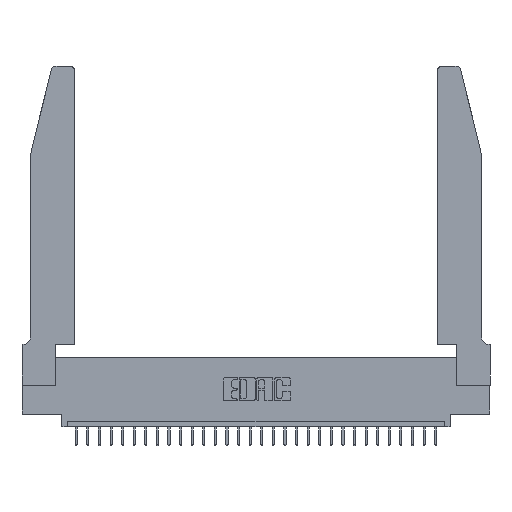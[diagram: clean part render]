
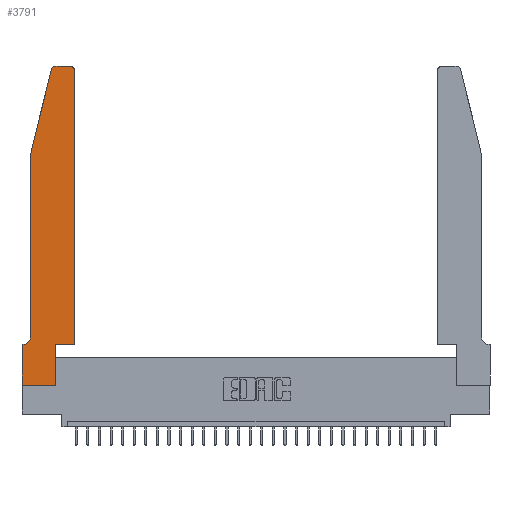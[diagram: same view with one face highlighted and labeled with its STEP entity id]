
A CAD part, top view. The second image highlights one B-rep face of the part: STEP entity #3791.
In plain terms, the highlighted planar face has unit normal (0, 0, 1).
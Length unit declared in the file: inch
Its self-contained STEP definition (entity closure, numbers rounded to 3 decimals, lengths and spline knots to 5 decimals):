
#134 = VECTOR ( 'NONE', #1609, 39.37008 ) ;
#528 = DIRECTION ( 'NONE',  ( 0., 0., 1. ) ) ;
#985 = DIRECTION ( 'NONE',  ( -1., 0., 0. ) ) ;
#990 = ORIENTED_EDGE ( 'NONE', *, *, #5058, .T. ) ;
#1609 = DIRECTION ( 'NONE',  ( 1., 0., 0. ) ) ;
#1809 = VECTOR ( 'NONE', #11846, 39.37008 ) ;
#2272 = EDGE_CURVE ( 'NONE', #11705, #8610, #29116, .T. ) ;
#2925 = VECTOR ( 'NONE', #13264, 39.37008 ) ;
#3066 = VECTOR ( 'NONE', #985, 39.37008 ) ;
#3258 = VERTEX_POINT ( 'NONE', #20159 ) ;
#3511 = ORIENTED_EDGE ( 'NONE', *, *, #26599, .T. ) ;
#3589 = ORIENTED_EDGE ( 'NONE', *, *, #25843, .T. ) ;
#3628 = EDGE_CURVE ( 'NONE', #18461, #7957, #4170, .T. ) ;
#3791 = ADVANCED_FACE ( 'NONE', ( #6734 ), #9200, .T. ) ;
#4170 = LINE ( 'NONE', #5717, #134 ) ;
#4307 = VECTOR ( 'NONE', #5583, 39.37008 ) ;
#5058 = EDGE_CURVE ( 'NONE', #7957, #29282, #20505, .T. ) ;
#5583 = DIRECTION ( 'NONE',  ( 0., -1., 0. ) ) ;
#5599 = EDGE_CURVE ( 'NONE', #6334, #9313, #20091, .T. ) ;
#5654 = DIRECTION ( 'NONE',  ( 0., 1., 0. ) ) ;
#5717 = CARTESIAN_POINT ( 'NONE',  ( 0.4505, 0.35, 0.37 ) ) ;
#6334 = VERTEX_POINT ( 'NONE', #29637 ) ;
#6403 = CARTESIAN_POINT ( 'NONE',  ( 0.0755, 2., 0.37 ) ) ;
#6659 = EDGE_CURVE ( 'NONE', #3258, #16181, #11992, .T. ) ;
#6734 = FACE_OUTER_BOUND ( 'NONE', #21080, .T. ) ;
#7278 = DIRECTION ( 'NONE',  ( 0., 0., -1. ) ) ;
#7701 = CARTESIAN_POINT ( 'NONE',  ( 0.0055, 0.42, 0.37 ) ) ;
#7957 = VERTEX_POINT ( 'NONE', #18358 ) ;
#8610 = VERTEX_POINT ( 'NONE', #6403 ) ;
#8666 = ORIENTED_EDGE ( 'NONE', *, *, #18599, .T. ) ;
#8841 = CARTESIAN_POINT ( 'NONE',  ( 0.0755, 2., 0.37 ) ) ;
#8984 = CARTESIAN_POINT ( 'NONE',  ( 0.4505, 2.72, 0.37 ) ) ;
#9177 = ORIENTED_EDGE ( 'NONE', *, *, #10182, .T. ) ;
#9200 = PLANE ( 'NONE',  #27149 ) ;
#9276 = DIRECTION ( 'NONE',  ( -0.239, -0.971, 0. ) ) ;
#9313 = VERTEX_POINT ( 'NONE', #20942 ) ;
#10182 = EDGE_CURVE ( 'NONE', #17042, #10856, #27306, .T. ) ;
#10247 = LINE ( 'NONE', #25930, #1809 ) ;
#10289 = CARTESIAN_POINT ( 'NONE',  ( 0., 0., 0.37 ) ) ;
#10739 = CARTESIAN_POINT ( 'NONE',  ( 0.284, 2.75, 0.37 ) ) ;
#10856 = VERTEX_POINT ( 'NONE', #10739 ) ;
#11136 = AXIS2_PLACEMENT_3D ( 'NONE', #26828, #24238, #19478 ) ;
#11151 = VECTOR ( 'NONE', #14341, 39.37008 ) ;
#11296 = VERTEX_POINT ( 'NONE', #16465 ) ;
#11705 = VERTEX_POINT ( 'NONE', #14014 ) ;
#11846 = DIRECTION ( 'NONE',  ( 0., 1., 0. ) ) ;
#11992 = CIRCLE ( 'NONE', #22037, 0.07 ) ;
#12599 = ORIENTED_EDGE ( 'NONE', *, *, #22833, .T. ) ;
#12634 = ORIENTED_EDGE ( 'NONE', *, *, #19811, .T. ) ;
#13264 = DIRECTION ( 'NONE',  ( 1., 0., 0. ) ) ;
#13458 = ORIENTED_EDGE ( 'NONE', *, *, #6659, .T. ) ;
#14014 = CARTESIAN_POINT ( 'NONE',  ( 0.25487, 2.72718, 0.37 ) ) ;
#14341 = DIRECTION ( 'NONE',  ( -1., 0., 0. ) ) ;
#14538 = CARTESIAN_POINT ( 'NONE',  ( 0.284, 2.72, 0.37 ) ) ;
#15014 = AXIS2_PLACEMENT_3D ( 'NONE', #14538, #528, #16856 ) ;
#15079 = CARTESIAN_POINT ( 'NONE',  ( 0.0755, 0.35, 0.37 ) ) ;
#15454 = DIRECTION ( 'NONE',  ( 0., -1., 0. ) ) ;
#16181 = VERTEX_POINT ( 'NONE', #18975 ) ;
#16263 = DIRECTION ( 'NONE',  ( -1., 0., 0. ) ) ;
#16465 = CARTESIAN_POINT ( 'NONE',  ( 0., 0.35, 0.37 ) ) ;
#16856 = DIRECTION ( 'NONE',  ( 1., 0., 0. ) ) ;
#17042 = VERTEX_POINT ( 'NONE', #28911 ) ;
#17098 = ORIENTED_EDGE ( 'NONE', *, *, #2272, .T. ) ;
#17205 = VECTOR ( 'NONE', #5654, 39.37008 ) ;
#17458 = ORIENTED_EDGE ( 'NONE', *, *, #5599, .T. ) ;
#17671 = LINE ( 'NONE', #15079, #3066 ) ;
#18071 = CIRCLE ( 'NONE', #15014, 0.03 ) ;
#18225 = ORIENTED_EDGE ( 'NONE', *, *, #21415, .T. ) ;
#18358 = CARTESIAN_POINT ( 'NONE',  ( 0.4505, 0.35, 0.37 ) ) ;
#18461 = VERTEX_POINT ( 'NONE', #21506 ) ;
#18599 = EDGE_CURVE ( 'NONE', #11296, #6334, #20736, .T. ) ;
#18975 = CARTESIAN_POINT ( 'NONE',  ( 0.0055, 0.35, 0.37 ) ) ;
#19478 = DIRECTION ( 'NONE',  ( 1., 0., 0. ) ) ;
#19811 = EDGE_CURVE ( 'NONE', #10856, #11705, #18071, .T. ) ;
#20091 = LINE ( 'NONE', #27334, #2925 ) ;
#20159 = CARTESIAN_POINT ( 'NONE',  ( 0.0755, 0.42, 0.37 ) ) ;
#20505 = LINE ( 'NONE', #24992, #17205 ) ;
#20736 = LINE ( 'NONE', #10289, #4307 ) ;
#20942 = CARTESIAN_POINT ( 'NONE',  ( 0.2865, 0., 0.37 ) ) ;
#21080 = EDGE_LOOP ( 'NONE', ( #9177, #12634, #17098, #3589, #13458, #3511, #8666, #17458, #12599, #23591, #990, #18225 ) ) ;
#21415 = EDGE_CURVE ( 'NONE', #29282, #17042, #22825, .T. ) ;
#21506 = CARTESIAN_POINT ( 'NONE',  ( 0.2865, 0.35, 0.37 ) ) ;
#22037 = AXIS2_PLACEMENT_3D ( 'NONE', #7701, #7278, #16263 ) ;
#22543 = LINE ( 'NONE', #8841, #26603 ) ;
#22825 = CIRCLE ( 'NONE', #11136, 0.03 ) ;
#22833 = EDGE_CURVE ( 'NONE', #9313, #18461, #10247, .T. ) ;
#22835 = VECTOR ( 'NONE', #9276, 39.37008 ) ;
#23591 = ORIENTED_EDGE ( 'NONE', *, *, #3628, .T. ) ;
#24238 = DIRECTION ( 'NONE',  ( 0., 0., 1. ) ) ;
#24992 = CARTESIAN_POINT ( 'NONE',  ( 0.4505, 0.35, 0.37 ) ) ;
#25791 = CARTESIAN_POINT ( 'NONE',  ( 0., 0.35, 0.37 ) ) ;
#25843 = EDGE_CURVE ( 'NONE', #8610, #3258, #22543, .T. ) ;
#25930 = CARTESIAN_POINT ( 'NONE',  ( 0.2865, 0.35, 0.37 ) ) ;
#26599 = EDGE_CURVE ( 'NONE', #16181, #11296, #17671, .T. ) ;
#26603 = VECTOR ( 'NONE', #15454, 39.37008 ) ;
#26828 = CARTESIAN_POINT ( 'NONE',  ( 0.4205, 2.72, 0.37 ) ) ;
#27149 = AXIS2_PLACEMENT_3D ( 'NONE', #25791, #30416, #27842 ) ;
#27306 = LINE ( 'NONE', #28437, #11151 ) ;
#27334 = CARTESIAN_POINT ( 'NONE',  ( 0., 0., 0.37 ) ) ;
#27842 = DIRECTION ( 'NONE',  ( 1., 0., 0. ) ) ;
#28019 = CARTESIAN_POINT ( 'NONE',  ( 0.0755, 2., 0.37 ) ) ;
#28437 = CARTESIAN_POINT ( 'NONE',  ( 0.2605, 2.75, 0.37 ) ) ;
#28911 = CARTESIAN_POINT ( 'NONE',  ( 0.4205, 2.75, 0.37 ) ) ;
#29116 = LINE ( 'NONE', #28019, #22835 ) ;
#29282 = VERTEX_POINT ( 'NONE', #8984 ) ;
#29637 = CARTESIAN_POINT ( 'NONE',  ( 0., 0., 0.37 ) ) ;
#30416 = DIRECTION ( 'NONE',  ( 0., 0., 1. ) ) ;
